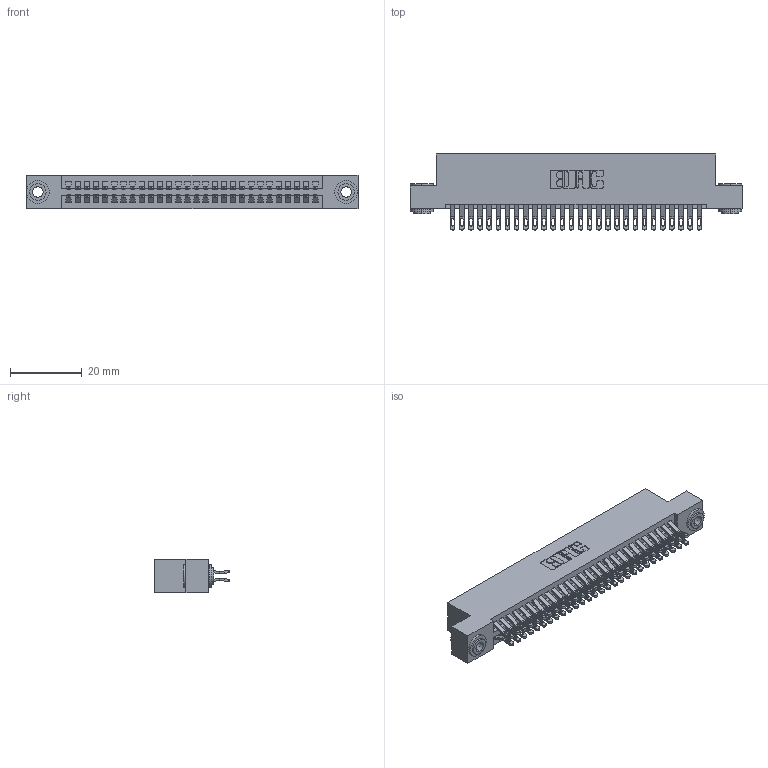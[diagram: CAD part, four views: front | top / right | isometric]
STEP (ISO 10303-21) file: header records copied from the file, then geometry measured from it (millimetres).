
FILE_DESCRIPTION (( 'STEP AP203' ), '1' );
FILE_NAME ('395-056-555-203.STEP', '2018-11-22T05:43:59', ( '' ), ( '' ), 'SwSTEP 2.0', 'SolidWorks 2016', '' );
FILE_SCHEMA (( 'CONFIG_CONTROL_DESIGN' ));
Length unit declared in the file: inch
Products named in the file (4): 345-292-001_555 Tail; 395-056-555-203; 345-250-002_345-250-002-102; 345 Part_Flush Mounting Lugs - 0.156 Dia-TH
Assembly tree (59 placements, depth 2):
  395-056-555-203
    345 Part_Flush Mounting Lugs - 0.156 Dia-TH
    345-292-001_555 Tail  x56
    345-250-002_345-250-002-102  x2
Bounding box: 92.33 x 21.13 x 9.4 mm (x, y, z)
Volume: 9020.8 mm3; surface area: 13833 mm2
Topology: 59 solids, 59 shells, 3300 faces, 10329 edges, 6882 vertices
Faces by surface type: plane 1826, cylinder 1466, cone 8
Entity records: 24830 total; most frequent: CARTESIAN_POINT 4185, ORIENTED_EDGE 4082, DIRECTION 3707, EDGE_CURVE 2041, LINE 1753, VECTOR 1753, VERTEX_POINT 1358, AXIS2_PLACEMENT_3D 977
